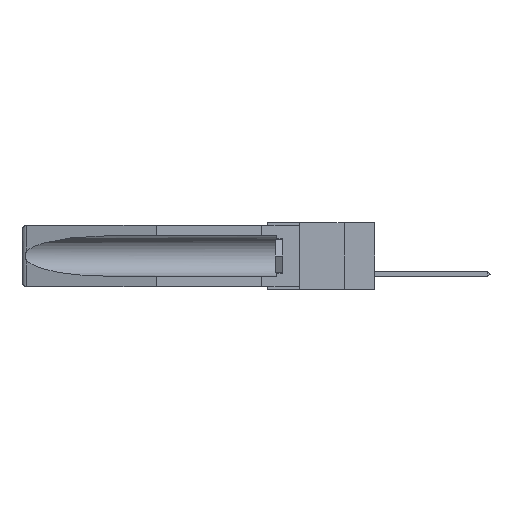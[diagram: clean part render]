
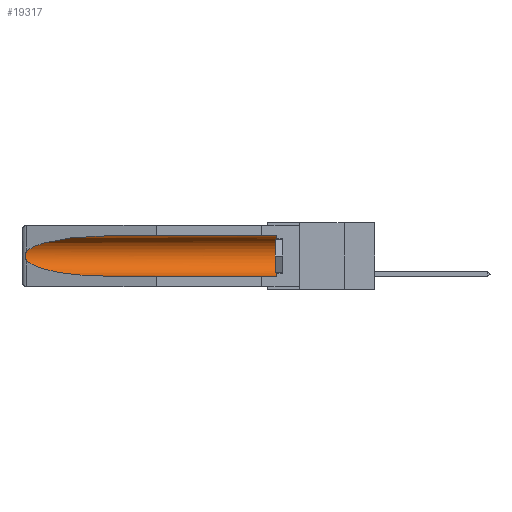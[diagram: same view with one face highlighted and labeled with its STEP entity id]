
A CAD part, left-side view. The second image highlights one B-rep face of the part: STEP entity #19317.
In plain terms, the highlighted cylindrical face has radius 2.857 mm (diameter 5.715 mm), a partial arc.
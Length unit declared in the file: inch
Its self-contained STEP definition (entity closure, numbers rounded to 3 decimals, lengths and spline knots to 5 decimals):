
#66 = CIRCLE ( 'NONE', #1301, 0.1125 ) ;
#151 = CARTESIAN_POINT ( 'NONE',  ( 0.2673, 1.53269, -0.17917 ) ) ;
#329 = VECTOR ( 'NONE', #10375, 39.37008 ) ;
#333 = EDGE_CURVE ( 'NONE', #6488, #5248, #13818, .T. ) ;
#1144 = CARTESIAN_POINT ( 'NONE',  ( 0.26537, 1.52718, -0.14972 ) ) ;
#1301 = AXIS2_PLACEMENT_3D ( 'NONE', #15982, #21027, #14074 ) ;
#1335 = EDGE_CURVE ( 'NONE', #8783, #3068, #66, .T. ) ;
#1715 = CARTESIAN_POINT ( 'NONE',  ( 0.2675, 1.53308, -0.16763 ) ) ;
#1926 = CARTESIAN_POINT ( 'NONE',  ( 0.155, 1.07973, -0.284 ) ) ;
#3068 = VERTEX_POINT ( 'NONE', #6254 ) ;
#3308 = CARTESIAN_POINT ( 'NONE',  ( 0.26654, 1.53092, -0.15636 ) ) ;
#3549 = ORIENTED_EDGE ( 'NONE', *, *, #1335, .T. ) ;
#5025 = LINE ( 'NONE', #18721, #329 ) ;
#5182 = CARTESIAN_POINT ( 'NONE',  ( 0.26597, 1.52961, -0.15275 ) ) ;
#5248 = VERTEX_POINT ( 'NONE', #22712 ) ;
#6232 = EDGE_CURVE ( 'NONE', #8783, #5248, #15701, .T. ) ;
#6254 = CARTESIAN_POINT ( 'NONE',  ( 0.155, 0.126, -0.059 ) ) ;
#6488 = VERTEX_POINT ( 'NONE', #9452 ) ;
#6892 = FACE_OUTER_BOUND ( 'NONE', #9246, .T. ) ;
#7155 = CARTESIAN_POINT ( 'NONE',  ( 0.26537, 1.52718, -0.19328 ) ) ;
#7279 = CARTESIAN_POINT ( 'NONE',  ( 0.155, -0.30754, -0.284 ) ) ;
#7400 = CARTESIAN_POINT ( 'NONE',  ( 0.26537, 1.52718, -0.14972 ) ) ;
#8059 = AXIS2_PLACEMENT_3D ( 'NONE', #18716, #13575, #20462 ) ;
#8145 = CARTESIAN_POINT ( 'NONE',  ( 0.25451, 1.48313, -0.09465 ) ) ;
#8610 = CARTESIAN_POINT ( 'NONE',  ( 0.155, 0.126, -0.284 ) ) ;
#8783 = VERTEX_POINT ( 'NONE', #8610 ) ;
#9246 = EDGE_LOOP ( 'NONE', ( #20939, #22049, #13611, #22775, #3549, #17712 ) ) ;
#9452 = CARTESIAN_POINT ( 'NONE',  ( 0.26537, 1.52718, -0.19328 ) ) ;
#9724 = EDGE_CURVE ( 'NONE', #11598, #16548, #10452, .T. ) ;
#10375 = DIRECTION ( 'NONE',  ( 0., 1., 0. ) ) ;
#10452 =( BOUNDED_CURVE ( )  B_SPLINE_CURVE ( 3, ( #13759, #22179, #8145, #1144 ),
 .UNSPECIFIED., .F., .F. ) 
 B_SPLINE_CURVE_WITH_KNOTS ( ( 4, 4 ),
 ( 4.71239, 6.08839 ),
 .UNSPECIFIED. ) 
 CURVE ( )  GEOMETRIC_REPRESENTATION_ITEM ( )  RATIONAL_B_SPLINE_CURVE ( ( 1., 0.848, 0.848, 1. ) ) 
 REPRESENTATION_ITEM ( '' )  );
#11598 = VERTEX_POINT ( 'NONE', #11641 ) ;
#11641 = CARTESIAN_POINT ( 'NONE',  ( 0.155, 1.07973, -0.059 ) ) ;
#12629 = CARTESIAN_POINT ( 'NONE',  ( 0.26597, 1.5296, -0.19026 ) ) ;
#13575 = DIRECTION ( 'NONE',  ( 0., 1., 0. ) ) ;
#13611 = ORIENTED_EDGE ( 'NONE', *, *, #333, .T. ) ;
#13759 = CARTESIAN_POINT ( 'NONE',  ( 0.155, 1.07973, -0.059 ) ) ;
#13818 =( BOUNDED_CURVE ( )  B_SPLINE_CURVE ( 3, ( #7155, #21163, #21016, #1926 ),
 .UNSPECIFIED., .F., .T. ) 
 B_SPLINE_CURVE_WITH_KNOTS ( ( 4, 4 ),
 ( 0.1948, 1.5708 ),
 .UNSPECIFIED. ) 
 CURVE ( )  GEOMETRIC_REPRESENTATION_ITEM ( )  RATIONAL_B_SPLINE_CURVE ( ( 1., 0.848, 0.848, 1. ) ) 
 REPRESENTATION_ITEM ( '' )  );
#14027 = CARTESIAN_POINT ( 'NONE',  ( 0.2675, 1.53308, -0.17534 ) ) ;
#14074 = DIRECTION ( 'NONE',  ( 0., 0., 1. ) ) ;
#15701 = LINE ( 'NONE', #7279, #17603 ) ;
#15713 = EDGE_CURVE ( 'NONE', #3068, #11598, #5025, .T. ) ;
#15928 = CARTESIAN_POINT ( 'NONE',  ( 0.26537, 1.52718, -0.19328 ) ) ;
#15982 = CARTESIAN_POINT ( 'NONE',  ( 0.155, 0.126, -0.1715 ) ) ;
#16027 = DIRECTION ( 'NONE',  ( 0., 1., 0. ) ) ;
#16548 = VERTEX_POINT ( 'NONE', #7400 ) ;
#17603 = VECTOR ( 'NONE', #16027, 39.37008 ) ;
#17712 = ORIENTED_EDGE ( 'NONE', *, *, #15713, .T. ) ;
#17876 = B_SPLINE_CURVE_WITH_KNOTS ( 'NONE', 3,
 ( #20821, #5182, #3308, #20953, #1715, #14027, #151, #21426, #12629, #15928 ),
 .UNSPECIFIED., .F., .F.,
 ( 4, 2, 2, 2, 4 ),
 ( 0., 0.00029, 0.00058, 0.00087, 0.00117 ),
 .UNSPECIFIED. ) ;
#18716 = CARTESIAN_POINT ( 'NONE',  ( 0.155, -0.30754, -0.1715 ) ) ;
#18721 = CARTESIAN_POINT ( 'NONE',  ( 0.155, -0.30754, -0.059 ) ) ;
#19317 = ADVANCED_FACE ( 'NONE', ( #6892 ), #21985, .F. ) ;
#20061 = EDGE_CURVE ( 'NONE', #16548, #6488, #17876, .T. ) ;
#20462 = DIRECTION ( 'NONE',  ( 0., 0., 1. ) ) ;
#20821 = CARTESIAN_POINT ( 'NONE',  ( 0.26537, 1.52718, -0.14972 ) ) ;
#20939 = ORIENTED_EDGE ( 'NONE', *, *, #9724, .T. ) ;
#20953 = CARTESIAN_POINT ( 'NONE',  ( 0.2673, 1.5327, -0.16383 ) ) ;
#21016 = CARTESIAN_POINT ( 'NONE',  ( 0.21114, 1.30732, -0.284 ) ) ;
#21027 = DIRECTION ( 'NONE',  ( 0., -1., 0. ) ) ;
#21163 = CARTESIAN_POINT ( 'NONE',  ( 0.25451, 1.48313, -0.24835 ) ) ;
#21426 = CARTESIAN_POINT ( 'NONE',  ( 0.26655, 1.53094, -0.18657 ) ) ;
#21985 = CYLINDRICAL_SURFACE ( 'NONE', #8059, 0.1125 ) ;
#22049 = ORIENTED_EDGE ( 'NONE', *, *, #20061, .T. ) ;
#22179 = CARTESIAN_POINT ( 'NONE',  ( 0.21114, 1.30732, -0.059 ) ) ;
#22712 = CARTESIAN_POINT ( 'NONE',  ( 0.155, 1.07973, -0.284 ) ) ;
#22775 = ORIENTED_EDGE ( 'NONE', *, *, #6232, .F. ) ;
